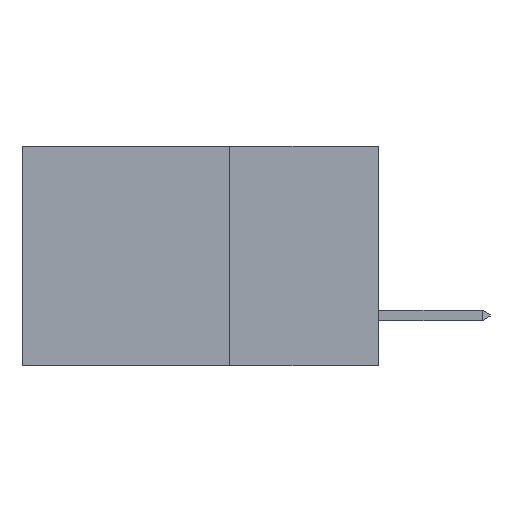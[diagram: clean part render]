
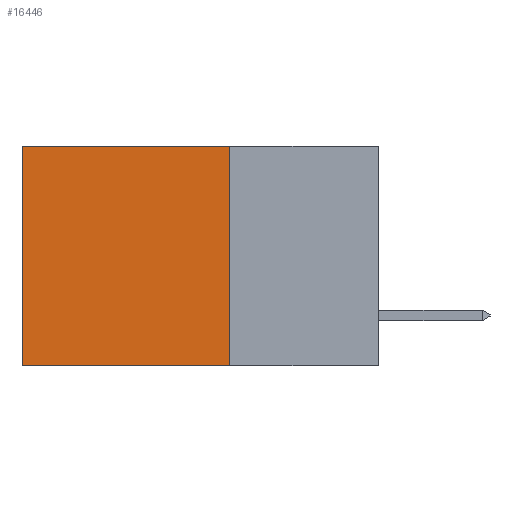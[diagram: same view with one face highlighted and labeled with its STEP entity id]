
A CAD part, left-side view. The second image highlights one B-rep face of the part: STEP entity #16446.
In plain terms, the highlighted planar face has unit normal (-1, 0, 0).
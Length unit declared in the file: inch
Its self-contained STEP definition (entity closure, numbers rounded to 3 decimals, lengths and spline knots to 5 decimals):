
#416 = ORIENTED_EDGE ( 'NONE', *, *, #14669, .T. ) ;
#517 = VECTOR ( 'NONE', #12776, 39.37008 ) ;
#887 = CARTESIAN_POINT ( 'NONE',  ( 0.298, 0.25, -0.37 ) ) ;
#959 = LINE ( 'NONE', #5095, #18629 ) ;
#1536 = CARTESIAN_POINT ( 'NONE',  ( 0.298, 0.25, 0. ) ) ;
#1705 = FACE_OUTER_BOUND ( 'NONE', #21586, .T. ) ;
#3203 = ORIENTED_EDGE ( 'NONE', *, *, #14286, .F. ) ;
#3556 = CARTESIAN_POINT ( 'NONE',  ( 0.298, 0.6, 0. ) ) ;
#3905 = CARTESIAN_POINT ( 'NONE',  ( 0.298, 0.25, 0. ) ) ;
#4067 = CARTESIAN_POINT ( 'NONE',  ( 0.298, 0.6, -0.37 ) ) ;
#4182 = VERTEX_POINT ( 'NONE', #887 ) ;
#5095 = CARTESIAN_POINT ( 'NONE',  ( 0.298, 0.25, 0. ) ) ;
#5774 = DIRECTION ( 'NONE',  ( 0., 0., -1. ) ) ;
#6351 = CARTESIAN_POINT ( 'NONE',  ( 0.298, 0.25, -0.37 ) ) ;
#8484 = VERTEX_POINT ( 'NONE', #1536 ) ;
#8846 = EDGE_CURVE ( 'NONE', #4182, #23222, #16377, .T. ) ;
#10290 = LINE ( 'NONE', #15266, #19147 ) ;
#10455 = LINE ( 'NONE', #3556, #517 ) ;
#11273 = EDGE_CURVE ( 'NONE', #20707, #23222, #10455, .T. ) ;
#11673 = VECTOR ( 'NONE', #20682, 39.37008 ) ;
#12776 = DIRECTION ( 'NONE',  ( 0., 0., -1. ) ) ;
#14286 = EDGE_CURVE ( 'NONE', #8484, #4182, #959, .T. ) ;
#14669 = EDGE_CURVE ( 'NONE', #8484, #20707, #10290, .T. ) ;
#15266 = CARTESIAN_POINT ( 'NONE',  ( 0.298, 0.25, 0. ) ) ;
#16377 = LINE ( 'NONE', #6351, #11673 ) ;
#16446 = ADVANCED_FACE ( 'NONE', ( #1705 ), #21808, .F. ) ;
#16635 = DIRECTION ( 'NONE',  ( 1., 0., 0. ) ) ;
#17764 = DIRECTION ( 'NONE',  ( 0., 0., -1. ) ) ;
#18465 = AXIS2_PLACEMENT_3D ( 'NONE', #3905, #16635, #5774 ) ;
#18629 = VECTOR ( 'NONE', #17764, 39.37008 ) ;
#18816 = DIRECTION ( 'NONE',  ( 0., 1., 0. ) ) ;
#19147 = VECTOR ( 'NONE', #18816, 39.37008 ) ;
#20438 = ORIENTED_EDGE ( 'NONE', *, *, #8846, .F. ) ;
#20682 = DIRECTION ( 'NONE',  ( 0., 1., 0. ) ) ;
#20707 = VERTEX_POINT ( 'NONE', #21812 ) ;
#21586 = EDGE_LOOP ( 'NONE', ( #23099, #20438, #3203, #416 ) ) ;
#21808 = PLANE ( 'NONE',  #18465 ) ;
#21812 = CARTESIAN_POINT ( 'NONE',  ( 0.298, 0.6, 0. ) ) ;
#23099 = ORIENTED_EDGE ( 'NONE', *, *, #11273, .T. ) ;
#23222 = VERTEX_POINT ( 'NONE', #4067 ) ;
